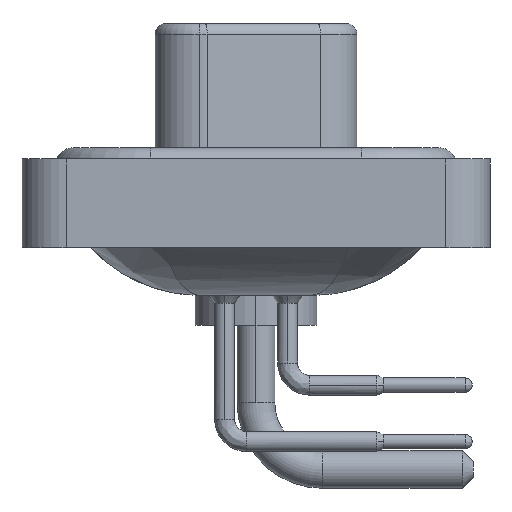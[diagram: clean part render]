
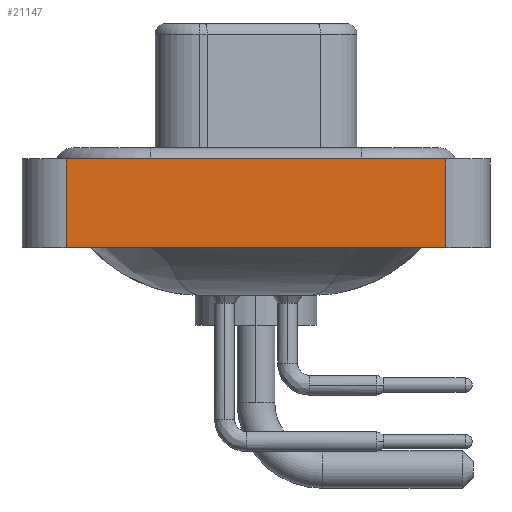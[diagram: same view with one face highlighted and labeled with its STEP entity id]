
A CAD part, left-side view. The second image highlights one B-rep face of the part: STEP entity #21147.
In plain terms, the highlighted planar face has unit normal (-1, 0, 0).
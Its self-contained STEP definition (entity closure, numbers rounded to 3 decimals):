
#219 = FACE_OUTER_BOUND ( 'NONE', #11924, .T. ) ;
#1267 = CARTESIAN_POINT ( 'NONE',  ( -7.25, -8.55, 0.4 ) ) ;
#3564 = CARTESIAN_POINT ( 'NONE',  ( -7.25, -8.55, 0.4 ) ) ;
#3661 = CARTESIAN_POINT ( 'NONE',  ( -7.25, 8.55, 0.4 ) ) ;
#4003 = DIRECTION ( 'NONE',  ( -1., 0., 0. ) ) ;
#4132 = CARTESIAN_POINT ( 'NONE',  ( -7.25, -8.55, -3.6 ) ) ;
#4364 = CARTESIAN_POINT ( 'NONE',  ( -7.25, 8.55, -3.6 ) ) ;
#4846 = LINE ( 'NONE', #8085, #6623 ) ;
#5970 = ORIENTED_EDGE ( 'NONE', *, *, #19161, .T. ) ;
#6134 = ORIENTED_EDGE ( 'NONE', *, *, #10019, .F. ) ;
#6623 = VECTOR ( 'NONE', #13618, 1000. ) ;
#6757 = DIRECTION ( 'NONE',  ( 0., 0., 1. ) ) ;
#6935 = VERTEX_POINT ( 'NONE', #3661 ) ;
#7149 = CARTESIAN_POINT ( 'NONE',  ( -7.25, -8.55, -3.6 ) ) ;
#7448 = VECTOR ( 'NONE', #17530, 1000. ) ;
#7589 = CARTESIAN_POINT ( 'NONE',  ( -7.25, 8.55, -3.6 ) ) ;
#8030 = ORIENTED_EDGE ( 'NONE', *, *, #10788, .T. ) ;
#8085 = CARTESIAN_POINT ( 'NONE',  ( -7.25, -8.55, -3.6 ) ) ;
#9298 = AXIS2_PLACEMENT_3D ( 'NONE', #7149, #4003, #16240 ) ;
#9587 = VERTEX_POINT ( 'NONE', #1267 ) ;
#10019 = EDGE_CURVE ( 'NONE', #12020, #6935, #16837, .T. ) ;
#10281 = LINE ( 'NONE', #21124, #17623 ) ;
#10788 = EDGE_CURVE ( 'NONE', #19169, #9587, #4846, .T. ) ;
#11906 = EDGE_CURVE ( 'NONE', #6935, #9587, #19373, .T. ) ;
#11924 = EDGE_LOOP ( 'NONE', ( #8030, #14306, #6134, #5970 ) ) ;
#12020 = VERTEX_POINT ( 'NONE', #7589 ) ;
#13618 = DIRECTION ( 'NONE',  ( 0., 0., 1. ) ) ;
#13860 = DIRECTION ( 'NONE',  ( 0., -1., 0. ) ) ;
#14306 = ORIENTED_EDGE ( 'NONE', *, *, #11906, .F. ) ;
#16240 = DIRECTION ( 'NONE',  ( 0., 0., 1. ) ) ;
#16837 = LINE ( 'NONE', #4364, #18760 ) ;
#17530 = DIRECTION ( 'NONE',  ( 0., -1., 0. ) ) ;
#17623 = VECTOR ( 'NONE', #13860, 1000. ) ;
#18760 = VECTOR ( 'NONE', #6757, 1000. ) ;
#19161 = EDGE_CURVE ( 'NONE', #12020, #19169, #10281, .T. ) ;
#19169 = VERTEX_POINT ( 'NONE', #4132 ) ;
#19373 = LINE ( 'NONE', #3564, #7448 ) ;
#21124 = CARTESIAN_POINT ( 'NONE',  ( -7.25, -8.55, -3.6 ) ) ;
#21147 = ADVANCED_FACE ( 'NONE', ( #219 ), #21550, .T. ) ;
#21550 = PLANE ( 'NONE',  #9298 ) ;
